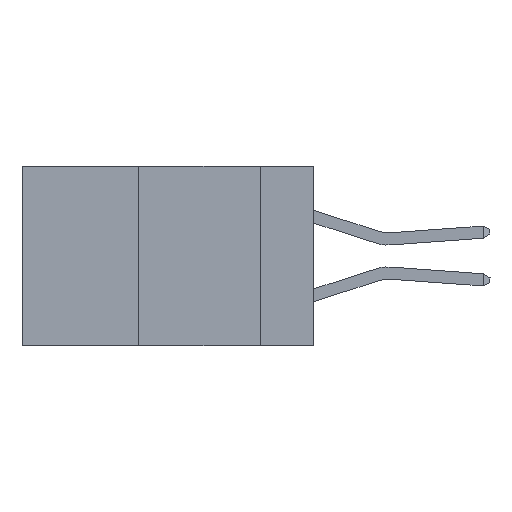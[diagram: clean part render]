
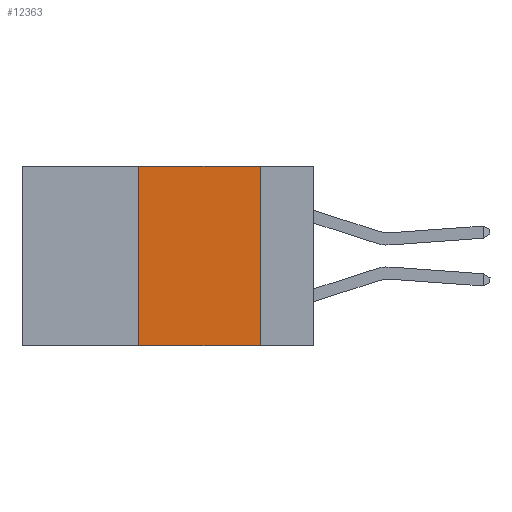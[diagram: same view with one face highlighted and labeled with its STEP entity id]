
A CAD part, left-side view. The second image highlights one B-rep face of the part: STEP entity #12363.
In plain terms, the highlighted planar face has unit normal (-1, 0, 0).
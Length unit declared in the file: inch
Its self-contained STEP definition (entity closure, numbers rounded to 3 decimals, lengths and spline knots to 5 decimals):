
#164 = LINE ( 'NONE', #4679, #6537 ) ;
#181 = DIRECTION ( 'NONE',  ( 0., 0., -1. ) ) ;
#233 = ORIENTED_EDGE ( 'NONE', *, *, #11024, .F. ) ;
#481 = EDGE_LOOP ( 'NONE', ( #6977, #233, #4088, #6049 ) ) ;
#1452 = DIRECTION ( 'NONE',  ( 0., -1., 0. ) ) ;
#2830 = VERTEX_POINT ( 'NONE', #11132 ) ;
#2946 = VERTEX_POINT ( 'NONE', #7903 ) ;
#3228 = CARTESIAN_POINT ( 'NONE',  ( 0., 0.11, -0.37 ) ) ;
#3383 = DIRECTION ( 'NONE',  ( 0., -1., 0. ) ) ;
#4063 = DIRECTION ( 'NONE',  ( 0., 0., 1. ) ) ;
#4088 = ORIENTED_EDGE ( 'NONE', *, *, #5198, .F. ) ;
#4273 = CARTESIAN_POINT ( 'NONE',  ( 0., 0.36, 0. ) ) ;
#4631 = LINE ( 'NONE', #6566, #8225 ) ;
#4679 = CARTESIAN_POINT ( 'NONE',  ( 0., 0.6, -0.37 ) ) ;
#5198 = EDGE_CURVE ( 'NONE', #2946, #2830, #14386, .T. ) ;
#5642 = VERTEX_POINT ( 'NONE', #14762 ) ;
#6049 = ORIENTED_EDGE ( 'NONE', *, *, #11343, .T. ) ;
#6523 = PLANE ( 'NONE',  #8541 ) ;
#6537 = VECTOR ( 'NONE', #3383, 39.37008 ) ;
#6566 = CARTESIAN_POINT ( 'NONE',  ( 0., 0.11, 0. ) ) ;
#6977 = ORIENTED_EDGE ( 'NONE', *, *, #11051, .F. ) ;
#7728 = DIRECTION ( 'NONE',  ( 1., 0., 0. ) ) ;
#7903 = CARTESIAN_POINT ( 'NONE',  ( 0., 0.36, -0.37 ) ) ;
#8202 = VECTOR ( 'NONE', #4063, 39.37008 ) ;
#8225 = VECTOR ( 'NONE', #14719, 39.37008 ) ;
#8541 = AXIS2_PLACEMENT_3D ( 'NONE', #13537, #7728, #181 ) ;
#9234 = VERTEX_POINT ( 'NONE', #3228 ) ;
#9972 = CARTESIAN_POINT ( 'NONE',  ( 0., 0.6, 0. ) ) ;
#10553 = FACE_OUTER_BOUND ( 'NONE', #481, .T. ) ;
#11024 = EDGE_CURVE ( 'NONE', #2830, #5642, #14404, .T. ) ;
#11051 = EDGE_CURVE ( 'NONE', #5642, #9234, #4631, .T. ) ;
#11132 = CARTESIAN_POINT ( 'NONE',  ( 0., 0.36, 0. ) ) ;
#11343 = EDGE_CURVE ( 'NONE', #2946, #9234, #164, .T. ) ;
#11345 = VECTOR ( 'NONE', #1452, 39.37008 ) ;
#12363 = ADVANCED_FACE ( 'NONE', ( #10553 ), #6523, .F. ) ;
#13537 = CARTESIAN_POINT ( 'NONE',  ( 0., 0.6, 0. ) ) ;
#14386 = LINE ( 'NONE', #4273, #8202 ) ;
#14404 = LINE ( 'NONE', #9972, #11345 ) ;
#14719 = DIRECTION ( 'NONE',  ( 0., 0., -1. ) ) ;
#14762 = CARTESIAN_POINT ( 'NONE',  ( 0., 0.11, 0. ) ) ;
